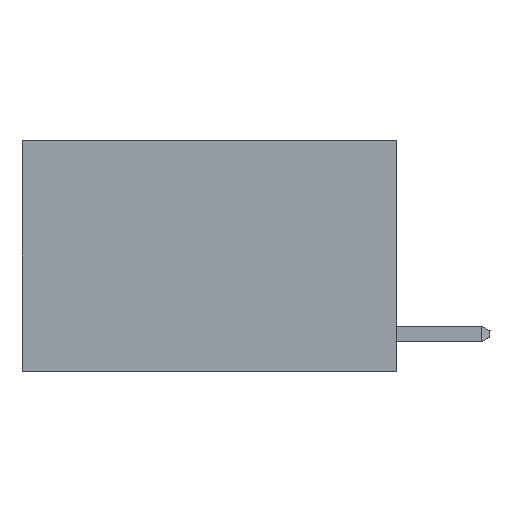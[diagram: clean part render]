
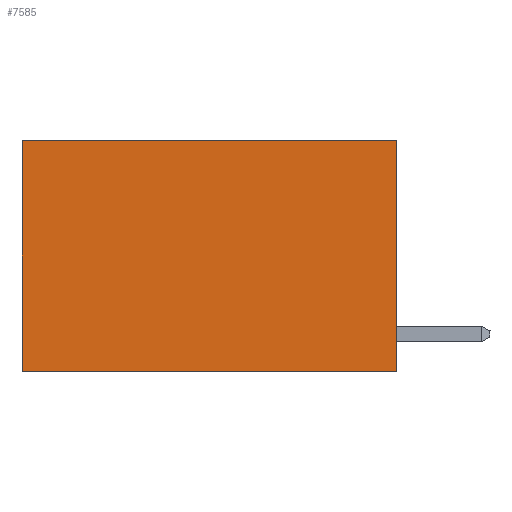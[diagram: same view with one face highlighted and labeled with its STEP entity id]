
A CAD part, left-side view. The second image highlights one B-rep face of the part: STEP entity #7585.
In plain terms, the highlighted planar face has unit normal (-1, 0, 0).
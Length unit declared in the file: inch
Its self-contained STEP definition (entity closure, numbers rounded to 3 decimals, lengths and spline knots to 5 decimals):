
#434 = VECTOR ( 'NONE', #9929, 39.37008 ) ;
#949 = VECTOR ( 'NONE', #3739, 39.37008 ) ;
#1373 = DIRECTION ( 'NONE',  ( 0., 0., -1. ) ) ;
#3147 = CARTESIAN_POINT ( 'NONE',  ( 0.2625, 0., 0. ) ) ;
#3739 = DIRECTION ( 'NONE',  ( 0., 1., 0. ) ) ;
#4423 = VERTEX_POINT ( 'NONE', #22903 ) ;
#4724 = ORIENTED_EDGE ( 'NONE', *, *, #13453, .F. ) ;
#6425 = LINE ( 'NONE', #3147, #434 ) ;
#6520 = DIRECTION ( 'NONE',  ( 1., 0., 0. ) ) ;
#7585 = ADVANCED_FACE ( 'NONE', ( #22559 ), #18074, .F. ) ;
#7972 = EDGE_CURVE ( 'NONE', #4423, #10857, #18670, .T. ) ;
#9207 = CARTESIAN_POINT ( 'NONE',  ( 0.2625, 0.6, 0. ) ) ;
#9224 = VERTEX_POINT ( 'NONE', #24526 ) ;
#9483 = ORIENTED_EDGE ( 'NONE', *, *, #20743, .F. ) ;
#9929 = DIRECTION ( 'NONE',  ( 0., 1., 0. ) ) ;
#10493 = LINE ( 'NONE', #21141, #18205 ) ;
#10857 = VERTEX_POINT ( 'NONE', #11465 ) ;
#11465 = CARTESIAN_POINT ( 'NONE',  ( 0.2625, 0.6, -0.37 ) ) ;
#13453 = EDGE_CURVE ( 'NONE', #24054, #10857, #21754, .T. ) ;
#13854 = ORIENTED_EDGE ( 'NONE', *, *, #7972, .T. ) ;
#14000 = EDGE_LOOP ( 'NONE', ( #13854, #4724, #9483, #25712 ) ) ;
#15902 = CARTESIAN_POINT ( 'NONE',  ( 0.2625, 0., 0. ) ) ;
#18074 = PLANE ( 'NONE',  #23711 ) ;
#18205 = VECTOR ( 'NONE', #1373, 39.37008 ) ;
#18670 = LINE ( 'NONE', #9207, #22200 ) ;
#19592 = CARTESIAN_POINT ( 'NONE',  ( 0.2625, 0., -0.37 ) ) ;
#20743 = EDGE_CURVE ( 'NONE', #9224, #24054, #10493, .T. ) ;
#21141 = CARTESIAN_POINT ( 'NONE',  ( 0.2625, 0., 0. ) ) ;
#21692 = CARTESIAN_POINT ( 'NONE',  ( 0.2625, 0., -0.37 ) ) ;
#21754 = LINE ( 'NONE', #21692, #949 ) ;
#22200 = VECTOR ( 'NONE', #22927, 39.37008 ) ;
#22310 = DIRECTION ( 'NONE',  ( 0., 0., -1. ) ) ;
#22559 = FACE_OUTER_BOUND ( 'NONE', #14000, .T. ) ;
#22903 = CARTESIAN_POINT ( 'NONE',  ( 0.2625, 0.6, 0. ) ) ;
#22920 = EDGE_CURVE ( 'NONE', #9224, #4423, #6425, .T. ) ;
#22927 = DIRECTION ( 'NONE',  ( 0., 0., -1. ) ) ;
#23711 = AXIS2_PLACEMENT_3D ( 'NONE', #15902, #6520, #22310 ) ;
#24054 = VERTEX_POINT ( 'NONE', #19592 ) ;
#24526 = CARTESIAN_POINT ( 'NONE',  ( 0.2625, 0., 0. ) ) ;
#25712 = ORIENTED_EDGE ( 'NONE', *, *, #22920, .T. ) ;
